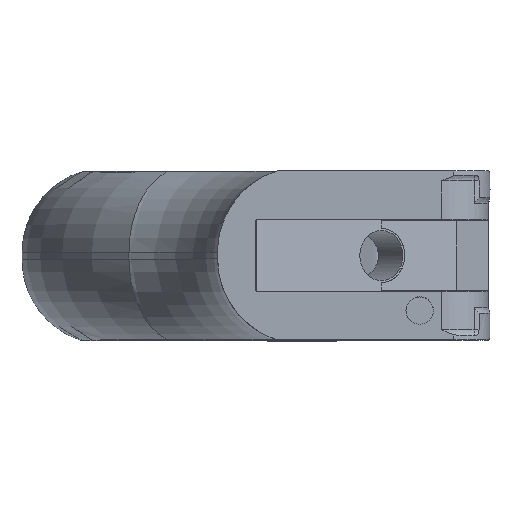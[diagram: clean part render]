
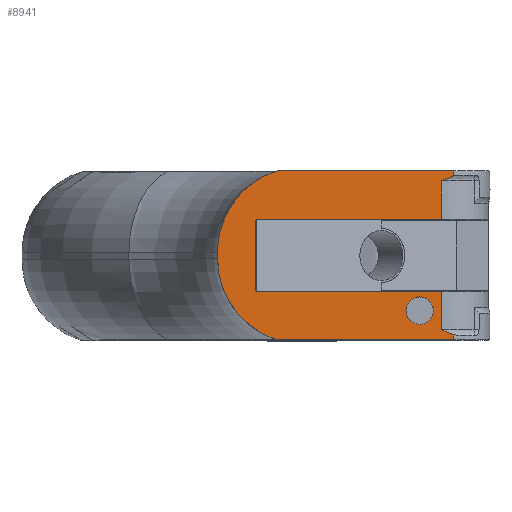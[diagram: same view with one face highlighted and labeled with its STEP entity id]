
A CAD part, top view. The second image highlights one B-rep face of the part: STEP entity #8941.
In plain terms, the highlighted planar face has unit normal (0.002, 0, 1).
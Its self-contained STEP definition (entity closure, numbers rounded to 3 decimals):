
#17=(
BOUNDED_CURVE()
B_SPLINE_CURVE(2,(#28665,#28666,#28667),.UNSPECIFIED.,.F.,.F.)
B_SPLINE_CURVE_WITH_KNOTS((3,3),(0.,2.53),
 .UNSPECIFIED.)
CURVE()
GEOMETRIC_REPRESENTATION_ITEM()
RATIONAL_B_SPLINE_CURVE((1.,0.993,1.))
REPRESENTATION_ITEM('')
);
#18=(
BOUNDED_CURVE()
B_SPLINE_CURVE(2,(#33838,#33839,#33840),.UNSPECIFIED.,.F.,.F.)
B_SPLINE_CURVE_WITH_KNOTS((3,3),(0.,2.53),.UNSPECIFIED.)
CURVE()
GEOMETRIC_REPRESENTATION_ITEM()
RATIONAL_B_SPLINE_CURVE((1.,0.993,1.))
REPRESENTATION_ITEM('')
);
#63=FACE_BOUND('',#3154,.T.);
#111=ELLIPSE('',#9264,11.57,11.57);
#112=ELLIPSE('',#9290,11.57,11.57);
#113=ELLIPSE('',#9291,1.875,1.875);
#157=PLANE('',#9289);
#1256=B_SPLINE_CURVE_WITH_KNOTS('',3,(#34364,#34365,#34366,#34367,#34368,
#34369),.UNSPECIFIED.,.F.,.F.,(4,2,4),(-0.142,0.,0.01),
 .UNSPECIFIED.);
#1260=B_SPLINE_CURVE_WITH_KNOTS('',3,(#37096,#37097,#37098,#37099),
 .UNSPECIFIED.,.F.,.F.,(4,4),(0.,0.161),
 .UNSPECIFIED.);
#1497=LINE('',#27540,#1947);
#1672=LINE('',#33848,#2122);
#1676=LINE('',#33856,#2126);
#1680=LINE('',#34160,#2130);
#1682=LINE('',#34206,#2132);
#1694=LINE('',#34278,#2144);
#1697=LINE('',#34321,#2147);
#1704=LINE('',#37080,#2154);
#1708=LINE('',#37088,#2158);
#1709=LINE('',#37093,#2159);
#1710=LINE('',#37094,#2160);
#1711=LINE('',#37095,#2161);
#1947=VECTOR('',#9985,10.);
#2122=VECTOR('',#10294,10.);
#2126=VECTOR('',#10300,10.);
#2130=VECTOR('',#10314,10.);
#2132=VECTOR('',#10322,10.);
#2144=VECTOR('',#10338,1.);
#2147=VECTOR('',#10353,1.);
#2154=VECTOR('',#10382,1.);
#2158=VECTOR('',#10394,1.);
#2159=VECTOR('',#10399,10.);
#2160=VECTOR('',#10400,10.);
#2161=VECTOR('',#10401,1.);
#2664=FACE_OUTER_BOUND('',#3153,.T.);
#3153=EDGE_LOOP('',(#8266,#8267,#8268,#8269,#8270,#8271,#8272,#8273,#8274,
#8275,#8276,#8277,#8278,#8279,#8280,#8281,#8282,#8283));
#3154=EDGE_LOOP('',(#8284));
#3963=VERTEX_POINT('',#27538);
#3964=VERTEX_POINT('',#27539);
#4093=VERTEX_POINT('',#28663);
#4094=VERTEX_POINT('',#28664);
#4228=VERTEX_POINT('',#33836);
#4229=VERTEX_POINT('',#33837);
#4230=VERTEX_POINT('',#33847);
#4233=VERTEX_POINT('',#33854);
#4241=VERTEX_POINT('',#34159);
#4245=VERTEX_POINT('',#34201);
#4246=VERTEX_POINT('',#34205);
#4256=VERTEX_POINT('',#34274);
#4258=VERTEX_POINT('',#34277);
#4262=VERTEX_POINT('',#34319);
#4268=VERTEX_POINT('',#34362);
#4269=VERTEX_POINT('',#34363);
#4272=VERTEX_POINT('',#37090);
#4273=VERTEX_POINT('',#37092);
#4274=VERTEX_POINT('',#37100);
#5142=EDGE_CURVE('',#3963,#3964,#1497,.T.);
#5285=EDGE_CURVE('',#4093,#4094,#17,.T.);
#5598=EDGE_CURVE('',#4228,#4229,#18,.T.);
#5601=EDGE_CURVE('',#4094,#4230,#1672,.T.);
#5605=EDGE_CURVE('',#4233,#4228,#1676,.T.);
#5617=EDGE_CURVE('',#4241,#3963,#1680,.T.);
#5622=EDGE_CURVE('',#3964,#4245,#111,.T.);
#5624=EDGE_CURVE('',#4246,#4245,#1682,.T.);
#5638=EDGE_CURVE('',#4258,#4256,#1694,.T.);
#5648=EDGE_CURVE('',#4262,#4093,#1697,.T.);
#5656=EDGE_CURVE('',#4268,#4269,#1256,.T.);
#5665=EDGE_CURVE('',#4233,#4258,#1704,.T.);
#5669=EDGE_CURVE('',#4229,#4269,#1708,.T.);
#5670=EDGE_CURVE('',#4246,#4272,#112,.T.);
#5671=EDGE_CURVE('',#4272,#4273,#1709,.T.);
#5672=EDGE_CURVE('',#4273,#4268,#1710,.T.);
#5673=EDGE_CURVE('',#4256,#4230,#1711,.T.);
#5674=EDGE_CURVE('',#4262,#4241,#1260,.T.);
#5675=EDGE_CURVE('',#4274,#4274,#113,.T.);
#8266=ORIENTED_EDGE('',*,*,#5670,.T.);
#8267=ORIENTED_EDGE('',*,*,#5671,.T.);
#8268=ORIENTED_EDGE('',*,*,#5672,.T.);
#8269=ORIENTED_EDGE('',*,*,#5656,.T.);
#8270=ORIENTED_EDGE('',*,*,#5669,.F.);
#8271=ORIENTED_EDGE('',*,*,#5598,.F.);
#8272=ORIENTED_EDGE('',*,*,#5605,.F.);
#8273=ORIENTED_EDGE('',*,*,#5665,.T.);
#8274=ORIENTED_EDGE('',*,*,#5638,.T.);
#8275=ORIENTED_EDGE('',*,*,#5673,.T.);
#8276=ORIENTED_EDGE('',*,*,#5601,.F.);
#8277=ORIENTED_EDGE('',*,*,#5285,.F.);
#8278=ORIENTED_EDGE('',*,*,#5648,.F.);
#8279=ORIENTED_EDGE('',*,*,#5674,.T.);
#8280=ORIENTED_EDGE('',*,*,#5617,.T.);
#8281=ORIENTED_EDGE('',*,*,#5142,.T.);
#8282=ORIENTED_EDGE('',*,*,#5622,.T.);
#8283=ORIENTED_EDGE('',*,*,#5624,.F.);
#8284=ORIENTED_EDGE('',*,*,#5675,.T.);
#8941=ADVANCED_FACE('',(#2664,#63),#157,.T.);
#9264=AXIS2_PLACEMENT_3D('',#34202,#10317,#10318);
#9289=AXIS2_PLACEMENT_3D('',#37089,#10395,#10396);
#9290=AXIS2_PLACEMENT_3D('',#37091,#10397,#10398);
#9291=AXIS2_PLACEMENT_3D('',#37101,#10402,#10403);
#9985=DIRECTION('',(-1.,0.,0.002));
#10294=DIRECTION('',(0.,-1.,0.));
#10300=DIRECTION('',(0.,-1.,0.));
#10314=DIRECTION('',(0.,1.,0.));
#10317=DIRECTION('center_axis',(0.002,0.,
1.));
#10318=DIRECTION('ref_axis',(-1.,0.,0.002));
#10322=DIRECTION('',(0.,1.,0.));
#10338=DIRECTION('',(0.,1.,0.));
#10353=DIRECTION('',(0.,-1.,0.));
#10382=DIRECTION('',(-1.,0.,0.002));
#10394=DIRECTION('',(0.,-1.,0.));
#10395=DIRECTION('center_axis',(0.002,0.,
1.));
#10396=DIRECTION('ref_axis',(0.711,-0.703,-0.001));
#10397=DIRECTION('center_axis',(0.002,0.,
1.));
#10398=DIRECTION('ref_axis',(-1.,0.,0.002));
#10399=DIRECTION('',(1.,0.,-0.002));
#10400=DIRECTION('',(0.,1.,0.));
#10401=DIRECTION('',(1.,0.,-0.002));
#10402=DIRECTION('center_axis',(-0.002,0.,
-1.));
#10403=DIRECTION('ref_axis',(1.,0.,-0.002));
#27538=CARTESIAN_POINT('',(2795.383,337.243,63.222));
#27539=CARTESIAN_POINT('',(2771.372,337.243,63.264));
#27540=CARTESIAN_POINT('',(2768.663,337.243,63.269));
#28663=CARTESIAN_POINT('',(2793.793,330.602,63.225));
#28664=CARTESIAN_POINT('',(2768.498,330.619,63.269));
#28665=CARTESIAN_POINT('Ctrl Pts',(2793.793,330.602,63.225));
#28666=CARTESIAN_POINT('Ctrl Pts',(2780.562,330.608,63.248));
#28667=CARTESIAN_POINT('Ctrl Pts',(2768.498,330.619,63.269));
#33836=CARTESIAN_POINT('',(2768.498,320.848,63.269));
#33837=CARTESIAN_POINT('',(2793.793,320.865,63.225));
#33838=CARTESIAN_POINT('Ctrl Pts',(2768.498,320.848,63.269));
#33839=CARTESIAN_POINT('Ctrl Pts',(2780.562,320.859,63.248));
#33840=CARTESIAN_POINT('Ctrl Pts',(2793.793,320.865,63.225));
#33847=CARTESIAN_POINT('',(2768.498,330.496,63.269));
#33848=CARTESIAN_POINT('',(2768.498,328.281,63.269));
#33854=CARTESIAN_POINT('',(2768.498,320.971,63.269));
#33856=CARTESIAN_POINT('',(2768.498,328.281,63.269));
#34159=CARTESIAN_POINT('',(2795.383,336.572,63.222));
#34160=CARTESIAN_POINT('',(2795.383,335.402,63.222));
#34201=CARTESIAN_POINT('',(2763.248,326.198,63.278));
#34202=CARTESIAN_POINT('Origin',(2774.818,326.198,63.258));
#34205=CARTESIAN_POINT('',(2763.248,325.278,63.278));
#34206=CARTESIAN_POINT('',(2763.248,317.109,63.278));
#34274=CARTESIAN_POINT('',(2768.393,330.496,63.269));
#34277=CARTESIAN_POINT('',(2768.393,320.971,63.269));
#34278=CARTESIAN_POINT('',(2768.393,322.527,63.269));
#34319=CARTESIAN_POINT('',(2793.793,335.894,63.225));
#34321=CARTESIAN_POINT('',(2793.793,335.519,63.225));
#34362=CARTESIAN_POINT('',(2795.383,314.896,63.222));
#34363=CARTESIAN_POINT('',(2793.793,315.574,63.225));
#34364=CARTESIAN_POINT('Ctrl Pts',(2795.383,314.896,63.222));
#34365=CARTESIAN_POINT('Ctrl Pts',(2794.837,315.106,63.223));
#34366=CARTESIAN_POINT('Ctrl Pts',(2794.319,315.339,63.224));
#34367=CARTESIAN_POINT('Ctrl Pts',(2793.855,315.546,63.225));
#34368=CARTESIAN_POINT('Ctrl Pts',(2793.839,315.553,63.225));
#34369=CARTESIAN_POINT('Ctrl Pts',(2793.793,315.574,63.225));
#37080=CARTESIAN_POINT('',(2791.345,320.971,63.229));
#37088=CARTESIAN_POINT('',(2793.793,318.839,63.225));
#37089=CARTESIAN_POINT('Origin',(2787.439,319.32,63.236));
#37090=CARTESIAN_POINT('',(2771.4,314.224,63.264));
#37091=CARTESIAN_POINT('Origin',(2774.818,325.278,63.258));
#37092=CARTESIAN_POINT('',(2795.383,314.224,63.222));
#37093=CARTESIAN_POINT('',(2768.663,314.224,63.269));
#37094=CARTESIAN_POINT('',(2795.383,316.065,63.222));
#37095=CARTESIAN_POINT('',(2791.345,330.496,63.229));
#37096=CARTESIAN_POINT('Ctrl Pts',(2793.793,335.894,63.225));
#37097=CARTESIAN_POINT('Ctrl Pts',(2794.283,336.113,63.224));
#37098=CARTESIAN_POINT('Ctrl Pts',(2794.843,336.364,63.223));
#37099=CARTESIAN_POINT('Ctrl Pts',(2795.383,336.572,63.222));
#37100=CARTESIAN_POINT('',(2788.895,318.215,63.234));
#37101=CARTESIAN_POINT('Origin',(2790.77,318.215,63.23));
